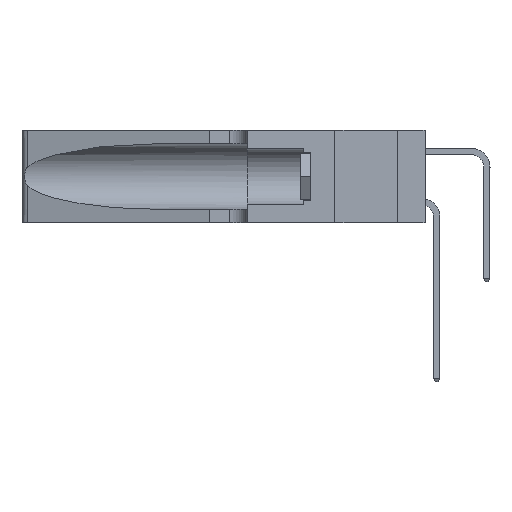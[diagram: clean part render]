
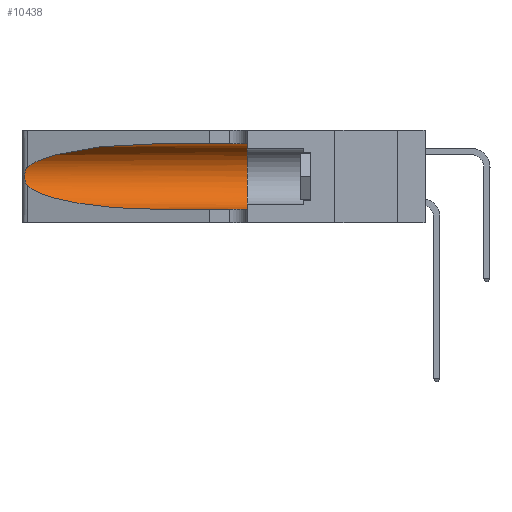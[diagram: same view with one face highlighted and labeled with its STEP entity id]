
A CAD part, left-side view. The second image highlights one B-rep face of the part: STEP entity #10438.
In plain terms, the highlighted cylindrical face has radius 3.308 mm (diameter 6.617 mm), a partial arc.
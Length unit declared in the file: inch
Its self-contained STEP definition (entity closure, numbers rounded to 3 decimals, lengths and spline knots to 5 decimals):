
#212 = CARTESIAN_POINT ( 'NONE',  ( 0.1305, 0.72297, 0.05475 ) ) ;
#403 = VECTOR ( 'NONE', #12939, 39.37008 ) ;
#665 = LINE ( 'NONE', #14836, #18936 ) ;
#1048 = CARTESIAN_POINT ( 'NONE',  ( 0.1305, 0.72297, 0.31525 ) ) ;
#1311 = CARTESIAN_POINT ( 'NONE',  ( 0.1305, 0.72297, 0.05475 ) ) ;
#1405 = CARTESIAN_POINT ( 'NONE',  ( 0.26075, 1.23896, 0.178 ) ) ;
#1540 = CIRCLE ( 'NONE', #2404, 0.13025 ) ;
#1695 = CARTESIAN_POINT ( 'NONE',  ( 0.26075, 1.23896, 0.19203 ) ) ;
#1762 = CARTESIAN_POINT ( 'NONE',  ( 0.25487, 1.22718, 0.14631 ) ) ;
#2319 = CYLINDRICAL_SURFACE ( 'NONE', #16011, 0.13025 ) ;
#2404 = AXIS2_PLACEMENT_3D ( 'NONE', #14022, #15972, #5824 ) ;
#2744 = EDGE_CURVE ( 'NONE', #7120, #20559, #665, .T. ) ;
#2862 = CARTESIAN_POINT ( 'NONE',  ( 0.2373, 1.15595, 0.28018 ) ) ;
#3039 = CARTESIAN_POINT ( 'NONE',  ( 0.1305, 1.61858, 0.185 ) ) ;
#3201 = CARTESIAN_POINT ( 'NONE',  ( 0.25787, 1.23484, 0.2124 ) ) ;
#4380 =( BOUNDED_CURVE ( )  B_SPLINE_CURVE ( 3, ( #1048, #17489, #2862, #19100 ),
 .UNSPECIFIED., .F., .F. ) 
 B_SPLINE_CURVE_WITH_KNOTS ( ( 4, 4 ),
 ( 1.5708, 2.84003 ),
 .UNSPECIFIED. ) 
 CURVE ( )  GEOMETRIC_REPRESENTATION_ITEM ( )  RATIONAL_B_SPLINE_CURVE ( ( 1., 0.87, 0.87, 1. ) ) 
 REPRESENTATION_ITEM ( '' )  );
#4620 = DIRECTION ( 'NONE',  ( 0., -1., 0. ) ) ;
#5824 = DIRECTION ( 'NONE',  ( 0., 0., 1. ) ) ;
#6690 = CARTESIAN_POINT ( 'NONE',  ( 0.1305, 0.35, 0.05475 ) ) ;
#7120 = VERTEX_POINT ( 'NONE', #16676 ) ;
#7967 = EDGE_CURVE ( 'NONE', #8036, #12686, #15884, .T. ) ;
#8026 = CARTESIAN_POINT ( 'NONE',  ( 0.26018, 1.23835, 0.19895 ) ) ;
#8036 = VERTEX_POINT ( 'NONE', #18032 ) ;
#8053 = DIRECTION ( 'NONE',  ( 0., -1., 0. ) ) ;
#8094 = CARTESIAN_POINT ( 'NONE',  ( 0.25789, 1.23486, 0.15765 ) ) ;
#9150 = LINE ( 'NONE', #16284, #403 ) ;
#9351 = EDGE_LOOP ( 'NONE', ( #18147, #9519, #13285, #12209, #17973, #15518 ) ) ;
#9519 = ORIENTED_EDGE ( 'NONE', *, *, #9939, .T. ) ;
#9575 = DIRECTION ( 'NONE',  ( 0., 0., -1. ) ) ;
#9609 = CARTESIAN_POINT ( 'NONE',  ( 0.25639, 1.23184, 0.21858 ) ) ;
#9939 = EDGE_CURVE ( 'NONE', #17188, #8036, #16529, .T. ) ;
#10438 = ADVANCED_FACE ( 'NONE', ( #17533 ), #2319, .F. ) ;
#11169 = CARTESIAN_POINT ( 'NONE',  ( 0.18966, 0.96281, 0.05475 ) ) ;
#11265 = CARTESIAN_POINT ( 'NONE',  ( 0.25854, 1.2359, 0.20912 ) ) ;
#11534 = CARTESIAN_POINT ( 'NONE',  ( 0.25487, 1.22718, 0.22369 ) ) ;
#12209 = ORIENTED_EDGE ( 'NONE', *, *, #19587, .T. ) ;
#12686 = VERTEX_POINT ( 'NONE', #212 ) ;
#12891 = CARTESIAN_POINT ( 'NONE',  ( 0.25856, 1.23593, 0.16098 ) ) ;
#12939 = DIRECTION ( 'NONE',  ( 0., -1., 0. ) ) ;
#13285 = ORIENTED_EDGE ( 'NONE', *, *, #7967, .T. ) ;
#13749 = CARTESIAN_POINT ( 'NONE',  ( 0.25487, 1.22718, 0.22369 ) ) ;
#14022 = CARTESIAN_POINT ( 'NONE',  ( 0.1305, 0.35, 0.185 ) ) ;
#14580 = CARTESIAN_POINT ( 'NONE',  ( 0.25555, 1.22993, 0.14849 ) ) ;
#14716 = CARTESIAN_POINT ( 'NONE',  ( 0.25639, 1.23186, 0.15144 ) ) ;
#14836 = CARTESIAN_POINT ( 'NONE',  ( 0.1305, 1.61858, 0.31525 ) ) ;
#14875 = CARTESIAN_POINT ( 'NONE',  ( 0.26017, 1.23833, 0.17102 ) ) ;
#14912 = EDGE_CURVE ( 'NONE', #7120, #17188, #4380, .T. ) ;
#15518 = ORIENTED_EDGE ( 'NONE', *, *, #2744, .F. ) ;
#15884 =( BOUNDED_CURVE ( )  B_SPLINE_CURVE ( 3, ( #1762, #17799, #11169, #1311 ),
 .UNSPECIFIED., .F., .F. ) 
 B_SPLINE_CURVE_WITH_KNOTS ( ( 4, 4 ),
 ( 3.44316, 4.71239 ),
 .UNSPECIFIED. ) 
 CURVE ( )  GEOMETRIC_REPRESENTATION_ITEM ( )  RATIONAL_B_SPLINE_CURVE ( ( 1., 0.87, 0.87, 1. ) ) 
 REPRESENTATION_ITEM ( '' )  );
#15972 = DIRECTION ( 'NONE',  ( 0., 1., 0. ) ) ;
#16011 = AXIS2_PLACEMENT_3D ( 'NONE', #3039, #4620, #9575 ) ;
#16284 = CARTESIAN_POINT ( 'NONE',  ( 0.1305, 1.61858, 0.05475 ) ) ;
#16385 = CARTESIAN_POINT ( 'NONE',  ( 0.25487, 1.22718, 0.14631 ) ) ;
#16529 = B_SPLINE_CURVE_WITH_KNOTS ( 'NONE', 3,
 ( #11534, #21101, #9609, #3201, #11265, #8026, #1695, #1405, #14875, #12891, #8094, #14716, #14580, #16385 ),
 .UNSPECIFIED., .F., .F.,
 ( 4, 2, 2, 2, 2, 2, 4 ),
 ( 0., 0.00027, 0.00053, 0.00107, 0.0016, 0.00187, 0.00214 ),
 .UNSPECIFIED. ) ;
#16567 = EDGE_CURVE ( 'NONE', #20559, #18008, #1540, .T. ) ;
#16676 = CARTESIAN_POINT ( 'NONE',  ( 0.1305, 0.72297, 0.31525 ) ) ;
#17188 = VERTEX_POINT ( 'NONE', #13749 ) ;
#17489 = CARTESIAN_POINT ( 'NONE',  ( 0.18966, 0.96281, 0.31525 ) ) ;
#17533 = FACE_OUTER_BOUND ( 'NONE', #9351, .T. ) ;
#17799 = CARTESIAN_POINT ( 'NONE',  ( 0.2373, 1.15595, 0.08982 ) ) ;
#17973 = ORIENTED_EDGE ( 'NONE', *, *, #16567, .F. ) ;
#18008 = VERTEX_POINT ( 'NONE', #6690 ) ;
#18032 = CARTESIAN_POINT ( 'NONE',  ( 0.25487, 1.22718, 0.14631 ) ) ;
#18147 = ORIENTED_EDGE ( 'NONE', *, *, #14912, .T. ) ;
#18936 = VECTOR ( 'NONE', #8053, 39.37008 ) ;
#19100 = CARTESIAN_POINT ( 'NONE',  ( 0.25487, 1.22718, 0.22369 ) ) ;
#19587 = EDGE_CURVE ( 'NONE', #12686, #18008, #9150, .T. ) ;
#20559 = VERTEX_POINT ( 'NONE', #20667 ) ;
#20667 = CARTESIAN_POINT ( 'NONE',  ( 0.1305, 0.35, 0.31525 ) ) ;
#21101 = CARTESIAN_POINT ( 'NONE',  ( 0.25555, 1.22994, 0.2215 ) ) ;
